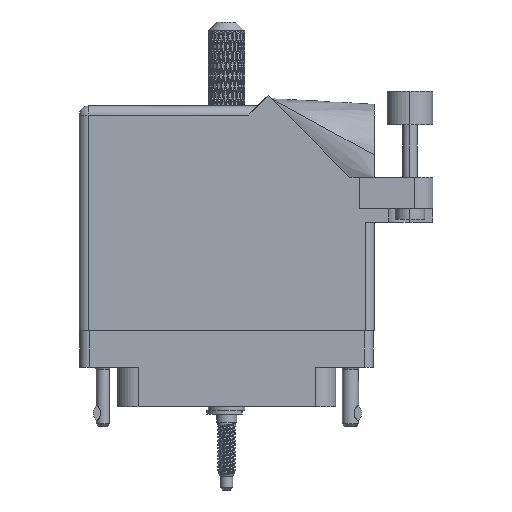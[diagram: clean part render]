
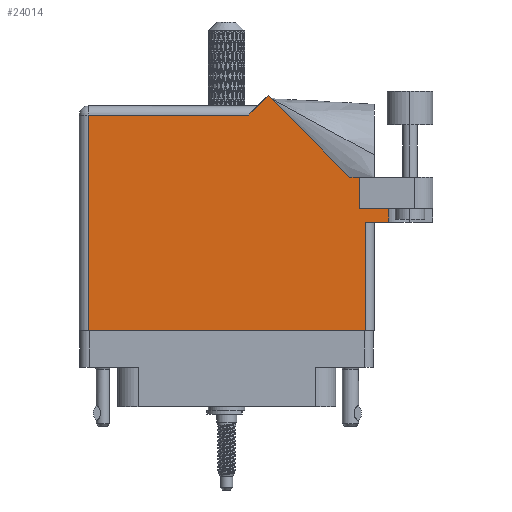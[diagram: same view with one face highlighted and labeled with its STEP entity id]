
A CAD part, front view. The second image highlights one B-rep face of the part: STEP entity #24014.
In plain terms, the highlighted face is planar.
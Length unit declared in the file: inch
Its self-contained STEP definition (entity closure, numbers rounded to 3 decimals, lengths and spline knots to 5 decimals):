
#1121 = DIRECTION ( 'NONE',  ( -0.707, -0.707, 0. ) ) ;
#1211 = ORIENTED_EDGE ( 'NONE', *, *, #87758, .T. ) ;
#2062 = EDGE_CURVE ( 'NONE', #64355, #33123, #94993, .T. ) ;
#4560 = ORIENTED_EDGE ( 'NONE', *, *, #101093, .T. ) ;
#4799 = DIRECTION ( 'NONE',  ( 0., -1., 0. ) ) ;
#5738 = CARTESIAN_POINT ( 'NONE',  ( -1.005, 1.368, 0.455 ) ) ;
#5922 = CARTESIAN_POINT ( 'NONE',  ( -1.005, -0.1, 0.455 ) ) ;
#9015 = EDGE_LOOP ( 'NONE', ( #17680, #84288, #97079, #80754, #49636, #1211, #4560, #11969, #71442, #83487, #48663 ) ) ;
#9038 = VERTEX_POINT ( 'NONE', #93813 ) ;
#11771 = CARTESIAN_POINT ( 'NONE',  ( -0.943, -0.1, 0.455 ) ) ;
#11969 = ORIENTED_EDGE ( 'NONE', *, *, #60565, .T. ) ;
#17164 = VECTOR ( 'NONE', #18270, 39.37008 ) ;
#17195 = CARTESIAN_POINT ( 'NONE',  ( 1.405, 0.944, 0.455 ) ) ;
#17480 = CARTESIAN_POINT ( 'NONE',  ( -0.943, 1.368, 0.455 ) ) ;
#17680 = ORIENTED_EDGE ( 'NONE', *, *, #88473, .T. ) ;
#17689 = CARTESIAN_POINT ( 'NONE',  ( 0.212, 1.43, 0.455 ) ) ;
#18270 = DIRECTION ( 'NONE',  ( 1., 0., 0. ) ) ;
#18390 = VERTEX_POINT ( 'NONE', #94254 ) ;
#21808 = VECTOR ( 'NONE', #90599, 39.37008 ) ;
#24014 = ADVANCED_FACE ( 'NONE', ( #63119 ), #91320, .F. ) ;
#25270 = VECTOR ( 'NONE', #40376, 39.37008 ) ;
#28342 = VERTEX_POINT ( 'NONE', #11771 ) ;
#30158 = VECTOR ( 'NONE', #44739, 39.37008 ) ;
#30636 = VERTEX_POINT ( 'NONE', #71786 ) ;
#30884 = EDGE_CURVE ( 'NONE', #30636, #63446, #89299, .T. ) ;
#33123 = VERTEX_POINT ( 'NONE', #68703 ) ;
#34635 = EDGE_CURVE ( 'NONE', #9038, #30636, #95965, .T. ) ;
#34971 = LINE ( 'NONE', #17195, #78035 ) ;
#35168 = CARTESIAN_POINT ( 'NONE',  ( 1.1065, 0.637, 0.455 ) ) ;
#35874 = VERTEX_POINT ( 'NONE', #44498 ) ;
#36450 = DIRECTION ( 'NONE',  ( 0., 1., 0. ) ) ;
#40376 = DIRECTION ( 'NONE',  ( -1., 0., 0. ) ) ;
#41249 = DIRECTION ( 'NONE',  ( 0., 0., -1. ) ) ;
#43656 = CARTESIAN_POINT ( 'NONE',  ( 0.905, 0.731, 0.455 ) ) ;
#44498 = CARTESIAN_POINT ( 'NONE',  ( 0.28271, 1.50071, 0.455 ) ) ;
#44683 = LINE ( 'NONE', #5922, #21808 ) ;
#44739 = DIRECTION ( 'NONE',  ( 1., 0., 0. ) ) ;
#45076 = LINE ( 'NONE', #77846, #108316 ) ;
#46210 = CARTESIAN_POINT ( 'NONE',  ( 0.905, 0.731, 0.455 ) ) ;
#48663 = ORIENTED_EDGE ( 'NONE', *, *, #50292, .T. ) ;
#49636 = ORIENTED_EDGE ( 'NONE', *, *, #34635, .F. ) ;
#50292 = EDGE_CURVE ( 'NONE', #64714, #28342, #45076, .T. ) ;
#51242 = LINE ( 'NONE', #79454, #64685 ) ;
#56422 = LINE ( 'NONE', #43656, #76565 ) ;
#60224 = LINE ( 'NONE', #61887, #17164 ) ;
#60565 = EDGE_CURVE ( 'NONE', #78363, #35874, #51242, .T. ) ;
#61887 = CARTESIAN_POINT ( 'NONE',  ( 1.005, 0.637, 0.455 ) ) ;
#63119 = FACE_OUTER_BOUND ( 'NONE', #9015, .T. ) ;
#63210 = VECTOR ( 'NONE', #1121, 39.37008 ) ;
#63446 = VERTEX_POINT ( 'NONE', #35168 ) ;
#64355 = VERTEX_POINT ( 'NONE', #78908 ) ;
#64685 = VECTOR ( 'NONE', #79817, 39.37008 ) ;
#64714 = VERTEX_POINT ( 'NONE', #17480 ) ;
#66377 = VECTOR ( 'NONE', #4799, 39.37008 ) ;
#68703 = CARTESIAN_POINT ( 'NONE',  ( 0.943, 0.637, 0.455 ) ) ;
#70462 = AXIS2_PLACEMENT_3D ( 'NONE', #99936, #41249, #102169 ) ;
#71442 = ORIENTED_EDGE ( 'NONE', *, *, #100736, .T. ) ;
#71786 = CARTESIAN_POINT ( 'NONE',  ( 1.1065, 0.731, 0.455 ) ) ;
#73398 = VECTOR ( 'NONE', #74395, 39.37008 ) ;
#74395 = DIRECTION ( 'NONE',  ( 0., 1., 0. ) ) ;
#76565 = VECTOR ( 'NONE', #36450, 39.37008 ) ;
#77846 = CARTESIAN_POINT ( 'NONE',  ( -0.943, -0.1, 0.455 ) ) ;
#78035 = VECTOR ( 'NONE', #103311, 39.37008 ) ;
#78363 = VERTEX_POINT ( 'NONE', #81231 ) ;
#78908 = CARTESIAN_POINT ( 'NONE',  ( 0.943, -0.1, 0.455 ) ) ;
#79454 = CARTESIAN_POINT ( 'NONE',  ( 0.83942, 0.944, 0.455 ) ) ;
#79817 = DIRECTION ( 'NONE',  ( -0.707, 0.707, 0. ) ) ;
#80754 = ORIENTED_EDGE ( 'NONE', *, *, #30884, .F. ) ;
#81231 = CARTESIAN_POINT ( 'NONE',  ( 0.83942, 0.944, 0.455 ) ) ;
#83115 = CARTESIAN_POINT ( 'NONE',  ( 1.1065, 1.06177, 0.455 ) ) ;
#83487 = ORIENTED_EDGE ( 'NONE', *, *, #108464, .T. ) ;
#84288 = ORIENTED_EDGE ( 'NONE', *, *, #2062, .T. ) ;
#84587 = LINE ( 'NONE', #5738, #25270 ) ;
#84863 = LINE ( 'NONE', #17689, #63210 ) ;
#85443 = VERTEX_POINT ( 'NONE', #86643 ) ;
#86643 = CARTESIAN_POINT ( 'NONE',  ( 0.15, 1.368, 0.455 ) ) ;
#87758 = EDGE_CURVE ( 'NONE', #9038, #18390, #56422, .T. ) ;
#88473 = EDGE_CURVE ( 'NONE', #28342, #64355, #44683, .T. ) ;
#89299 = LINE ( 'NONE', #83115, #66377 ) ;
#90599 = DIRECTION ( 'NONE',  ( 1., 0., 0. ) ) ;
#91320 = PLANE ( 'NONE',  #70462 ) ;
#92826 = CARTESIAN_POINT ( 'NONE',  ( 0.943, 0.637, 0.455 ) ) ;
#93813 = CARTESIAN_POINT ( 'NONE',  ( 0.905, 0.731, 0.455 ) ) ;
#94254 = CARTESIAN_POINT ( 'NONE',  ( 0.905, 0.944, 0.455 ) ) ;
#94392 = DIRECTION ( 'NONE',  ( 0., -1., 0. ) ) ;
#94993 = LINE ( 'NONE', #92826, #73398 ) ;
#95608 = EDGE_CURVE ( 'NONE', #33123, #63446, #60224, .T. ) ;
#95965 = LINE ( 'NONE', #46210, #30158 ) ;
#97079 = ORIENTED_EDGE ( 'NONE', *, *, #95608, .T. ) ;
#99936 = CARTESIAN_POINT ( 'NONE',  ( -1.005, 1.43, 0.455 ) ) ;
#100736 = EDGE_CURVE ( 'NONE', #35874, #85443, #84863, .T. ) ;
#101093 = EDGE_CURVE ( 'NONE', #18390, #78363, #34971, .T. ) ;
#102169 = DIRECTION ( 'NONE',  ( -1., 0., 0. ) ) ;
#103311 = DIRECTION ( 'NONE',  ( -1., 0., 0. ) ) ;
#108316 = VECTOR ( 'NONE', #94392, 39.37008 ) ;
#108464 = EDGE_CURVE ( 'NONE', #85443, #64714, #84587, .T. ) ;
